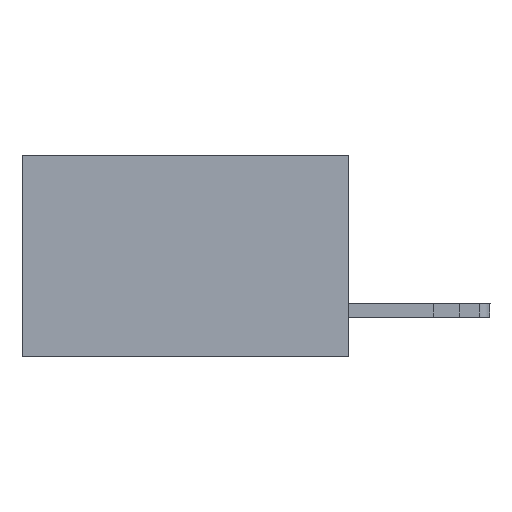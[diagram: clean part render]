
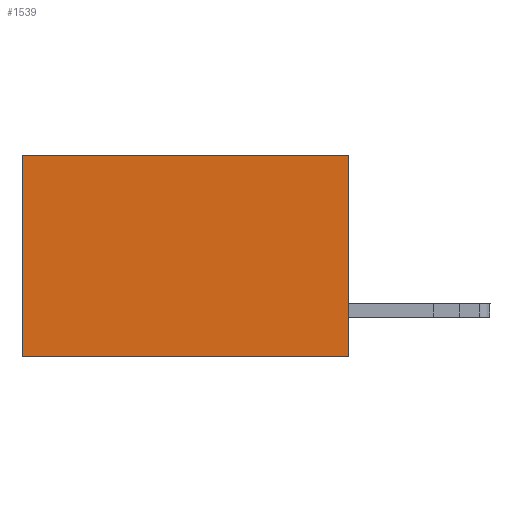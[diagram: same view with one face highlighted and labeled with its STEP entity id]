
A CAD part, left-side view. The second image highlights one B-rep face of the part: STEP entity #1539.
In plain terms, the highlighted planar face has unit normal (-1, 0, 0).
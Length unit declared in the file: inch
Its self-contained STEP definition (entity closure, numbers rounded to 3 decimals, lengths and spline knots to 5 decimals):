
#142 = LINE ( 'NONE', #2057, #5702 ) ;
#375 = EDGE_CURVE ( 'NONE', #2200, #2334, #9776, .T. ) ;
#537 = FACE_OUTER_BOUND ( 'NONE', #5709, .T. ) ;
#1539 = ADVANCED_FACE ( 'NONE', ( #537 ), #10895, .F. ) ;
#1826 = EDGE_CURVE ( 'NONE', #2290, #2245, #142, .T. ) ;
#1875 = EDGE_CURVE ( 'NONE', #2200, #2290, #6353, .T. ) ;
#2057 = CARTESIAN_POINT ( 'NONE',  ( 0.2615, 0., -0.37 ) ) ;
#2200 = VERTEX_POINT ( 'NONE', #11285 ) ;
#2245 = VERTEX_POINT ( 'NONE', #2326 ) ;
#2290 = VERTEX_POINT ( 'NONE', #9871 ) ;
#2326 = CARTESIAN_POINT ( 'NONE',  ( 0.2615, 0.6, -0.37 ) ) ;
#2334 = VERTEX_POINT ( 'NONE', #4291 ) ;
#2513 = ORIENTED_EDGE ( 'NONE', *, *, #1826, .F. ) ;
#2829 = ORIENTED_EDGE ( 'NONE', *, *, #375, .T. ) ;
#3009 = VECTOR ( 'NONE', #8547, 39.37008 ) ;
#4098 = ORIENTED_EDGE ( 'NONE', *, *, #1875, .F. ) ;
#4291 = CARTESIAN_POINT ( 'NONE',  ( 0.2615, 0.6, 0. ) ) ;
#4777 = LINE ( 'NONE', #6928, #8933 ) ;
#4925 = AXIS2_PLACEMENT_3D ( 'NONE', #11041, #10812, #10792 ) ;
#5251 = EDGE_CURVE ( 'NONE', #2334, #2245, #4777, .T. ) ;
#5702 = VECTOR ( 'NONE', #9549, 39.37008 ) ;
#5709 = EDGE_LOOP ( 'NONE', ( #7252, #2513, #4098, #2829 ) ) ;
#6353 = LINE ( 'NONE', #9948, #10567 ) ;
#6885 = DIRECTION ( 'NONE',  ( 0., 0., -1. ) ) ;
#6928 = CARTESIAN_POINT ( 'NONE',  ( 0.2615, 0.6, -0.37 ) ) ;
#7252 = ORIENTED_EDGE ( 'NONE', *, *, #5251, .T. ) ;
#8547 = DIRECTION ( 'NONE',  ( 0., 1., 0. ) ) ;
#8933 = VECTOR ( 'NONE', #6885, 39.37008 ) ;
#9549 = DIRECTION ( 'NONE',  ( 0., 1., 0. ) ) ;
#9776 = LINE ( 'NONE', #10565, #3009 ) ;
#9843 = DIRECTION ( 'NONE',  ( 0., 0., -1. ) ) ;
#9871 = CARTESIAN_POINT ( 'NONE',  ( 0.2615, 0., -0.37 ) ) ;
#9948 = CARTESIAN_POINT ( 'NONE',  ( 0.2615, 0., -0.37 ) ) ;
#10565 = CARTESIAN_POINT ( 'NONE',  ( 0.2615, 0., 0. ) ) ;
#10567 = VECTOR ( 'NONE', #9843, 39.37008 ) ;
#10792 = DIRECTION ( 'NONE',  ( 0., 0., -1. ) ) ;
#10812 = DIRECTION ( 'NONE',  ( 1., 0., 0. ) ) ;
#10895 = PLANE ( 'NONE',  #4925 ) ;
#11041 = CARTESIAN_POINT ( 'NONE',  ( 0.2615, 0., -0.37 ) ) ;
#11285 = CARTESIAN_POINT ( 'NONE',  ( 0.2615, 0., 0. ) ) ;
